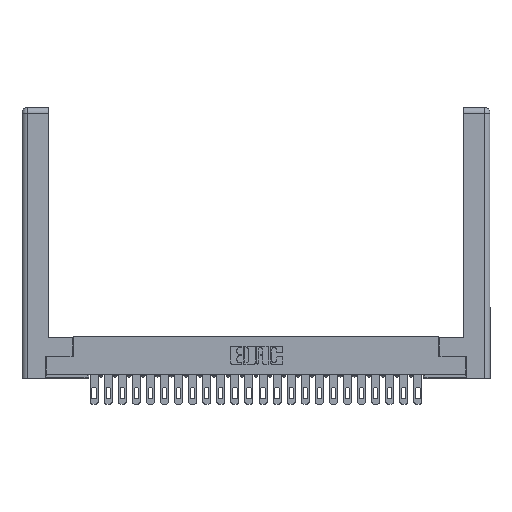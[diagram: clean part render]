
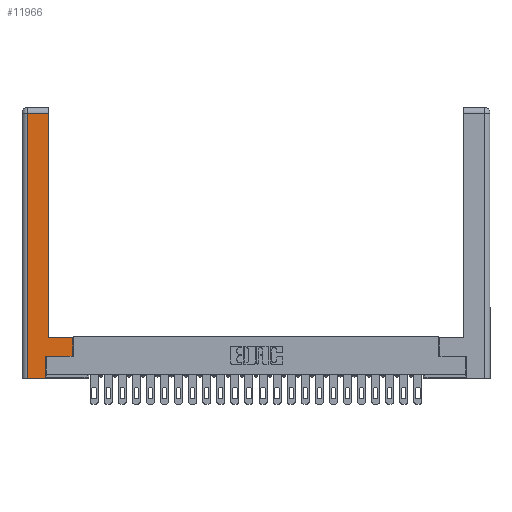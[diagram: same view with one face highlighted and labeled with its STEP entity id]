
A CAD part, top view. The second image highlights one B-rep face of the part: STEP entity #11966.
In plain terms, the highlighted planar face has unit normal (0, 0, 1).
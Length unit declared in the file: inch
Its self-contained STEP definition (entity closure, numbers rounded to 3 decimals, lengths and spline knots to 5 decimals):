
#873 = ORIENTED_EDGE ( 'NONE', *, *, #2846, .T. ) ;
#1532 = VERTEX_POINT ( 'NONE', #19258 ) ;
#1689 = VECTOR ( 'NONE', #18437, 39.37008 ) ;
#2385 = ORIENTED_EDGE ( 'NONE', *, *, #4626, .T. ) ;
#2686 = CARTESIAN_POINT ( 'NONE',  ( 0.0615, 2.94, 0. ) ) ;
#2846 = EDGE_CURVE ( 'NONE', #17949, #22156, #5660, .T. ) ;
#2991 = LINE ( 'NONE', #24579, #22193 ) ;
#3206 = LINE ( 'NONE', #19264, #16702 ) ;
#3550 = CARTESIAN_POINT ( 'NONE',  ( 0.295, 0.45, 0. ) ) ;
#3720 = VERTEX_POINT ( 'NONE', #17139 ) ;
#4175 = VERTEX_POINT ( 'NONE', #7978 ) ;
#4626 = EDGE_CURVE ( 'NONE', #10020, #3720, #24096, .T. ) ;
#5073 = AXIS2_PLACEMENT_3D ( 'NONE', #24560, #11191, #16970 ) ;
#5135 = VECTOR ( 'NONE', #10959, 39.37008 ) ;
#5660 = LINE ( 'NONE', #21306, #14995 ) ;
#6066 = EDGE_CURVE ( 'NONE', #24807, #4175, #7663, .T. ) ;
#6234 = CARTESIAN_POINT ( 'NONE',  ( 0.565, 0.245, 0. ) ) ;
#7663 = LINE ( 'NONE', #3550, #16101 ) ;
#7978 = CARTESIAN_POINT ( 'NONE',  ( 0.295, 0.45, 0. ) ) ;
#8399 = VECTOR ( 'NONE', #23598, 39.37008 ) ;
#8779 = EDGE_CURVE ( 'NONE', #4175, #16292, #3206, .T. ) ;
#10020 = VERTEX_POINT ( 'NONE', #10345 ) ;
#10175 = EDGE_CURVE ( 'NONE', #1532, #24807, #2991, .T. ) ;
#10345 = CARTESIAN_POINT ( 'NONE',  ( 0.265, 0., 0. ) ) ;
#10551 = VECTOR ( 'NONE', #19908, 39.37008 ) ;
#10843 = DIRECTION ( 'NONE',  ( 0., 1., 0. ) ) ;
#10959 = DIRECTION ( 'NONE',  ( 1., 0., 0. ) ) ;
#11054 = DIRECTION ( 'NONE',  ( 0., 1., 0. ) ) ;
#11191 = DIRECTION ( 'NONE',  ( 0., 0., -1. ) ) ;
#11552 = DIRECTION ( 'NONE',  ( 0., -1., 0. ) ) ;
#11966 = ADVANCED_FACE ( 'NONE', ( #13000 ), #22751, .F. ) ;
#12863 = EDGE_CURVE ( 'NONE', #3720, #1532, #17673, .T. ) ;
#13000 = FACE_OUTER_BOUND ( 'NONE', #21343, .T. ) ;
#13291 = ORIENTED_EDGE ( 'NONE', *, *, #13353, .T. ) ;
#13325 = DIRECTION ( 'NONE',  ( -1., 0., 0. ) ) ;
#13353 = EDGE_CURVE ( 'NONE', #22156, #10020, #18536, .T. ) ;
#14192 = CARTESIAN_POINT ( 'NONE',  ( 0.265, 0.245, 0. ) ) ;
#14995 = VECTOR ( 'NONE', #11552, 39.37008 ) ;
#15163 = ORIENTED_EDGE ( 'NONE', *, *, #12863, .T. ) ;
#15480 = CARTESIAN_POINT ( 'NONE',  ( 0.0615, 2.94, 0. ) ) ;
#15492 = CARTESIAN_POINT ( 'NONE',  ( 0.0615, 0., 0. ) ) ;
#16101 = VECTOR ( 'NONE', #13325, 39.37008 ) ;
#16292 = VERTEX_POINT ( 'NONE', #23301 ) ;
#16702 = VECTOR ( 'NONE', #11054, 39.37008 ) ;
#16970 = DIRECTION ( 'NONE',  ( -1., 0., 0. ) ) ;
#17139 = CARTESIAN_POINT ( 'NONE',  ( 0.265, 0.245, 0. ) ) ;
#17192 = EDGE_CURVE ( 'NONE', #16292, #17949, #21973, .T. ) ;
#17647 = ORIENTED_EDGE ( 'NONE', *, *, #6066, .T. ) ;
#17673 = LINE ( 'NONE', #6234, #8399 ) ;
#17949 = VERTEX_POINT ( 'NONE', #15480 ) ;
#18144 = ORIENTED_EDGE ( 'NONE', *, *, #10175, .T. ) ;
#18409 = CARTESIAN_POINT ( 'NONE',  ( 0.265, 0., 0. ) ) ;
#18437 = DIRECTION ( 'NONE',  ( 0., 1., 0. ) ) ;
#18536 = LINE ( 'NONE', #18409, #5135 ) ;
#19258 = CARTESIAN_POINT ( 'NONE',  ( 0.565, 0.245, 0. ) ) ;
#19264 = CARTESIAN_POINT ( 'NONE',  ( 0.295, 3., 0. ) ) ;
#19908 = DIRECTION ( 'NONE',  ( -1., 0., 0. ) ) ;
#21306 = CARTESIAN_POINT ( 'NONE',  ( 0.0615, 0., 0. ) ) ;
#21343 = EDGE_LOOP ( 'NONE', ( #25215, #23342, #873, #13291, #2385, #15163, #18144, #17647 ) ) ;
#21973 = LINE ( 'NONE', #2686, #10551 ) ;
#22156 = VERTEX_POINT ( 'NONE', #15492 ) ;
#22193 = VECTOR ( 'NONE', #10843, 39.37008 ) ;
#22383 = CARTESIAN_POINT ( 'NONE',  ( 0.565, 0.45, 0. ) ) ;
#22751 = PLANE ( 'NONE',  #5073 ) ;
#23301 = CARTESIAN_POINT ( 'NONE',  ( 0.295, 2.94, 0. ) ) ;
#23342 = ORIENTED_EDGE ( 'NONE', *, *, #17192, .T. ) ;
#23598 = DIRECTION ( 'NONE',  ( 1., 0., 0. ) ) ;
#24096 = LINE ( 'NONE', #14192, #1689 ) ;
#24560 = CARTESIAN_POINT ( 'NONE',  ( 0., 0., 0. ) ) ;
#24579 = CARTESIAN_POINT ( 'NONE',  ( 0.565, 0.45, 0. ) ) ;
#24807 = VERTEX_POINT ( 'NONE', #22383 ) ;
#25215 = ORIENTED_EDGE ( 'NONE', *, *, #8779, .T. ) ;
